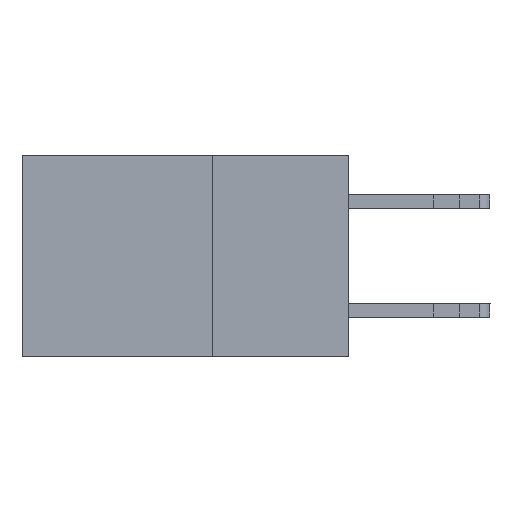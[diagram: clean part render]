
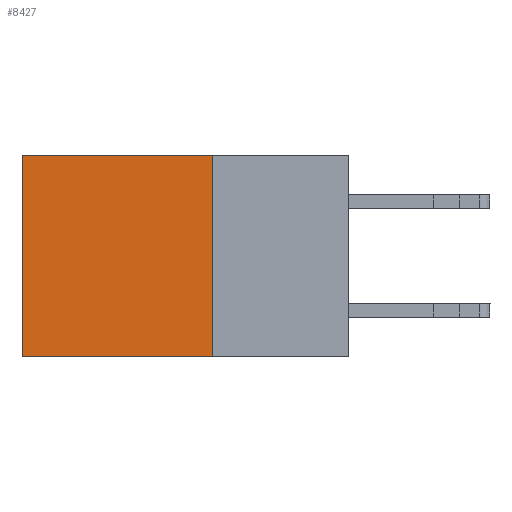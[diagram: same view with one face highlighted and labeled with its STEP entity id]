
A CAD part, left-side view. The second image highlights one B-rep face of the part: STEP entity #8427.
In plain terms, the highlighted planar face has unit normal (-1, 0, 0).
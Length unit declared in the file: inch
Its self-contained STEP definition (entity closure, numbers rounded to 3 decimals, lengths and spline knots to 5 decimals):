
#291 = AXIS2_PLACEMENT_3D ( 'NONE', #9683, #3621, #10676 ) ;
#569 = VECTOR ( 'NONE', #12669, 39.37008 ) ;
#820 = DIRECTION ( 'NONE',  ( 0., 0., -1. ) ) ;
#1160 = EDGE_CURVE ( 'NONE', #4873, #1524, #3309, .T. ) ;
#1524 = VERTEX_POINT ( 'NONE', #6499 ) ;
#1710 = LINE ( 'NONE', #7914, #7062 ) ;
#3309 = LINE ( 'NONE', #5254, #569 ) ;
#3621 = DIRECTION ( 'NONE',  ( 1., 0., 0. ) ) ;
#3693 = VECTOR ( 'NONE', #8152, 39.37008 ) ;
#3732 = VERTEX_POINT ( 'NONE', #4061 ) ;
#3883 = LINE ( 'NONE', #6124, #11301 ) ;
#4061 = CARTESIAN_POINT ( 'NONE',  ( 0.2615, 0.6, -0.37 ) ) ;
#4077 = ORIENTED_EDGE ( 'NONE', *, *, #12244, .F. ) ;
#4873 = VERTEX_POINT ( 'NONE', #10032 ) ;
#5151 = CARTESIAN_POINT ( 'NONE',  ( 0.2615, 0.6, -0.37 ) ) ;
#5254 = CARTESIAN_POINT ( 'NONE',  ( 0.2615, 0.25, 0. ) ) ;
#5345 = DIRECTION ( 'NONE',  ( 0., 1., 0. ) ) ;
#6124 = CARTESIAN_POINT ( 'NONE',  ( 0.2615, 0.25, -0.37 ) ) ;
#6165 = EDGE_LOOP ( 'NONE', ( #11499, #11827, #4077, #6819 ) ) ;
#6206 = VERTEX_POINT ( 'NONE', #12302 ) ;
#6499 = CARTESIAN_POINT ( 'NONE',  ( 0.2615, 0.6, 0. ) ) ;
#6819 = ORIENTED_EDGE ( 'NONE', *, *, #1160, .T. ) ;
#7062 = VECTOR ( 'NONE', #820, 39.37008 ) ;
#7077 = EDGE_CURVE ( 'NONE', #6206, #3732, #3883, .T. ) ;
#7656 = PLANE ( 'NONE',  #291 ) ;
#7914 = CARTESIAN_POINT ( 'NONE',  ( 0.2615, 0.25, -0.37 ) ) ;
#8152 = DIRECTION ( 'NONE',  ( 0., 0., -1. ) ) ;
#8427 = ADVANCED_FACE ( 'NONE', ( #10169 ), #7656, .F. ) ;
#8728 = EDGE_CURVE ( 'NONE', #1524, #3732, #9104, .T. ) ;
#9104 = LINE ( 'NONE', #5151, #3693 ) ;
#9683 = CARTESIAN_POINT ( 'NONE',  ( 0.2615, 0.25, -0.37 ) ) ;
#10032 = CARTESIAN_POINT ( 'NONE',  ( 0.2615, 0.25, 0. ) ) ;
#10169 = FACE_OUTER_BOUND ( 'NONE', #6165, .T. ) ;
#10676 = DIRECTION ( 'NONE',  ( 0., 0., -1. ) ) ;
#11301 = VECTOR ( 'NONE', #5345, 39.37008 ) ;
#11499 = ORIENTED_EDGE ( 'NONE', *, *, #8728, .T. ) ;
#11827 = ORIENTED_EDGE ( 'NONE', *, *, #7077, .F. ) ;
#12244 = EDGE_CURVE ( 'NONE', #4873, #6206, #1710, .T. ) ;
#12302 = CARTESIAN_POINT ( 'NONE',  ( 0.2615, 0.25, -0.37 ) ) ;
#12669 = DIRECTION ( 'NONE',  ( 0., 1., 0. ) ) ;
